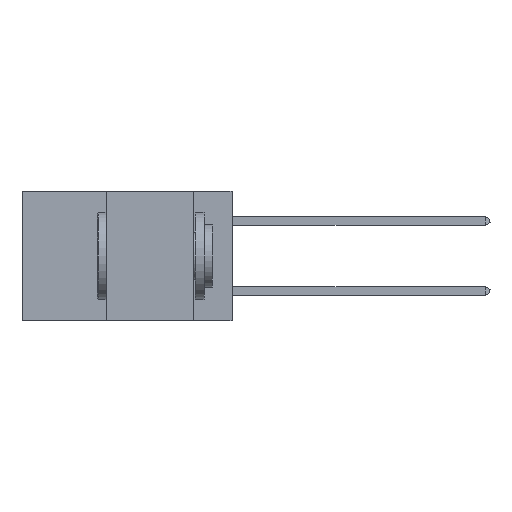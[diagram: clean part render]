
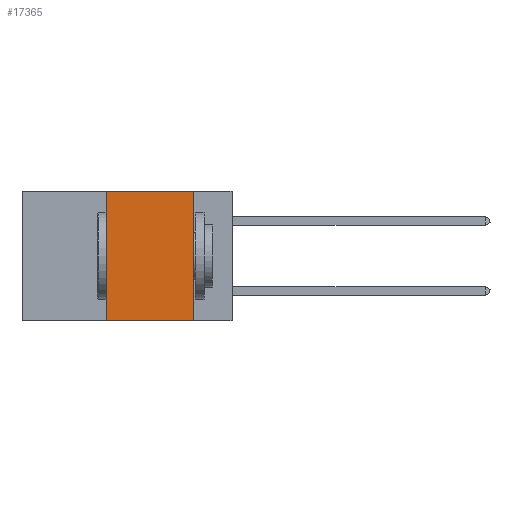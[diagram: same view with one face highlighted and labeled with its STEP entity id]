
A CAD part, left-side view. The second image highlights one B-rep face of the part: STEP entity #17365.
In plain terms, the highlighted planar face has unit normal (-1, 0, 0).
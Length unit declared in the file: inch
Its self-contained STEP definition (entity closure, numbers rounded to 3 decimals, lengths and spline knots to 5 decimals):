
#115 = CARTESIAN_POINT ( 'NONE',  ( 0., 0.11, 0. ) ) ;
#1667 = CARTESIAN_POINT ( 'NONE',  ( 0., 0.6, 0. ) ) ;
#3165 = CARTESIAN_POINT ( 'NONE',  ( 0., 0.6, -0.37 ) ) ;
#3519 = EDGE_LOOP ( 'NONE', ( #10818, #5093, #11591, #24961 ) ) ;
#3572 = CARTESIAN_POINT ( 'NONE',  ( 0., 0.11, -0.37 ) ) ;
#4320 = VECTOR ( 'NONE', #21749, 39.37008 ) ;
#5093 = ORIENTED_EDGE ( 'NONE', *, *, #11057, .F. ) ;
#5103 = VECTOR ( 'NONE', #5584, 39.37008 ) ;
#5584 = DIRECTION ( 'NONE',  ( 0., -1., 0. ) ) ;
#8685 = FACE_OUTER_BOUND ( 'NONE', #3519, .T. ) ;
#8867 = VERTEX_POINT ( 'NONE', #29135 ) ;
#9276 = LINE ( 'NONE', #115, #4320 ) ;
#9523 = CARTESIAN_POINT ( 'NONE',  ( 0., 0.36, 0. ) ) ;
#10617 = VERTEX_POINT ( 'NONE', #9523 ) ;
#10724 = EDGE_CURVE ( 'NONE', #22034, #17860, #9276, .T. ) ;
#10818 = ORIENTED_EDGE ( 'NONE', *, *, #10724, .F. ) ;
#10983 = CARTESIAN_POINT ( 'NONE',  ( 0., 0.6, 0. ) ) ;
#11057 = EDGE_CURVE ( 'NONE', #10617, #22034, #13039, .T. ) ;
#11591 = ORIENTED_EDGE ( 'NONE', *, *, #29380, .F. ) ;
#13039 = LINE ( 'NONE', #10983, #24896 ) ;
#13218 = VECTOR ( 'NONE', #28003, 39.37008 ) ;
#13888 = DIRECTION ( 'NONE',  ( 1., 0., 0. ) ) ;
#17365 = ADVANCED_FACE ( 'NONE', ( #8685 ), #28044, .F. ) ;
#17860 = VERTEX_POINT ( 'NONE', #3572 ) ;
#19543 = EDGE_CURVE ( 'NONE', #8867, #17860, #23492, .T. ) ;
#21749 = DIRECTION ( 'NONE',  ( 0., 0., -1. ) ) ;
#22034 = VERTEX_POINT ( 'NONE', #28481 ) ;
#23274 = CARTESIAN_POINT ( 'NONE',  ( 0., 0.36, 0. ) ) ;
#23492 = LINE ( 'NONE', #3165, #5103 ) ;
#24896 = VECTOR ( 'NONE', #27576, 39.37008 ) ;
#24961 = ORIENTED_EDGE ( 'NONE', *, *, #19543, .T. ) ;
#25811 = LINE ( 'NONE', #23274, #13218 ) ;
#26108 = AXIS2_PLACEMENT_3D ( 'NONE', #1667, #13888, #30390 ) ;
#27576 = DIRECTION ( 'NONE',  ( 0., -1., 0. ) ) ;
#28003 = DIRECTION ( 'NONE',  ( 0., 0., 1. ) ) ;
#28044 = PLANE ( 'NONE',  #26108 ) ;
#28481 = CARTESIAN_POINT ( 'NONE',  ( 0., 0.11, 0. ) ) ;
#29135 = CARTESIAN_POINT ( 'NONE',  ( 0., 0.36, -0.37 ) ) ;
#29380 = EDGE_CURVE ( 'NONE', #8867, #10617, #25811, .T. ) ;
#30390 = DIRECTION ( 'NONE',  ( 0., 0., -1. ) ) ;
